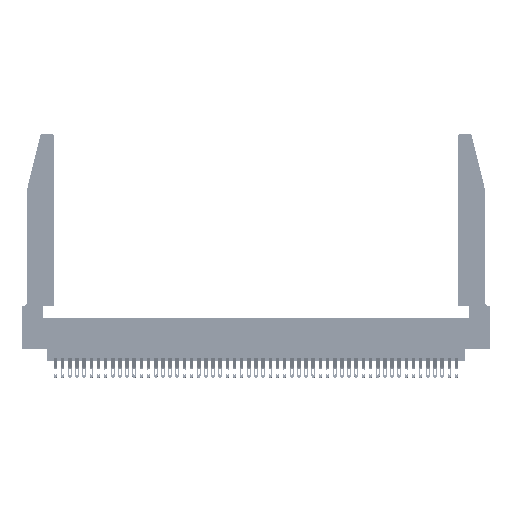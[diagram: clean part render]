
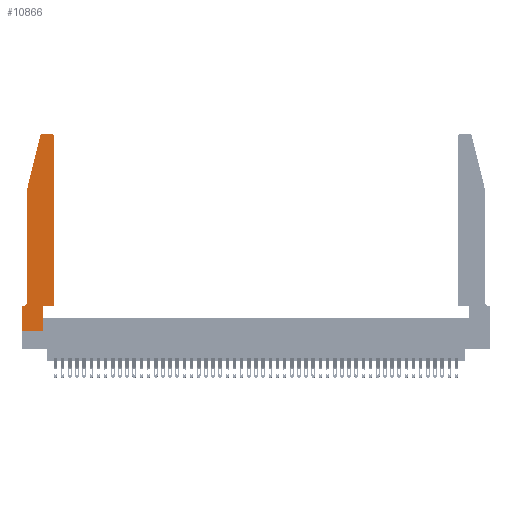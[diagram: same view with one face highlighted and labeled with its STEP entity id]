
A CAD part, top view. The second image highlights one B-rep face of the part: STEP entity #10866.
In plain terms, the highlighted planar face has unit normal (0, 0, 1).
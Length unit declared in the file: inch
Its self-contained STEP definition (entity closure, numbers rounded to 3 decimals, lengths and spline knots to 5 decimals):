
#9 = VERTEX_POINT ( 'NONE', #42469 ) ;
#34 = DIRECTION ( 'NONE',  ( 0., 0., -1. ) ) ;
#800 = LINE ( 'NONE', #43074, #20768 ) ;
#1021 = DIRECTION ( 'NONE',  ( 0., 1., 0. ) ) ;
#2736 = ORIENTED_EDGE ( 'NONE', *, *, #31449, .T. ) ;
#3164 = VERTEX_POINT ( 'NONE', #34432 ) ;
#3414 = VECTOR ( 'NONE', #1021, 39.37008 ) ;
#4061 = DIRECTION ( 'NONE',  ( 1., 0., 0. ) ) ;
#5102 = ORIENTED_EDGE ( 'NONE', *, *, #32296, .T. ) ;
#5123 = LINE ( 'NONE', #26429, #23848 ) ;
#5332 = VECTOR ( 'NONE', #27551, 39.37008 ) ;
#5709 = DIRECTION ( 'NONE',  ( 0., 0., 1. ) ) ;
#5745 = PLANE ( 'NONE',  #34677 ) ;
#5918 = DIRECTION ( 'NONE',  ( -1., 0., 0. ) ) ;
#5928 = CARTESIAN_POINT ( 'NONE',  ( 0.4205, 2.72, 0.37 ) ) ;
#7140 = ORIENTED_EDGE ( 'NONE', *, *, #41401, .T. ) ;
#7609 = EDGE_CURVE ( 'NONE', #45134, #28492, #46839, .T. ) ;
#7830 = CARTESIAN_POINT ( 'NONE',  ( 0., 0., 0.37 ) ) ;
#8157 = EDGE_CURVE ( 'NONE', #40730, #31751, #12805, .T. ) ;
#8918 = CARTESIAN_POINT ( 'NONE',  ( 0.2865, 0.35, 0.37 ) ) ;
#9130 = ORIENTED_EDGE ( 'NONE', *, *, #18466, .T. ) ;
#9181 = CARTESIAN_POINT ( 'NONE',  ( 0.4505, 0.35, 0.37 ) ) ;
#9729 = DIRECTION ( 'NONE',  ( 1., 0., 0. ) ) ;
#10556 = LINE ( 'NONE', #36836, #29129 ) ;
#10817 = ORIENTED_EDGE ( 'NONE', *, *, #7609, .T. ) ;
#10866 = ADVANCED_FACE ( 'NONE', ( #25432 ), #5745, .T. ) ;
#11307 = CARTESIAN_POINT ( 'NONE',  ( 0.0055, 0.35, 0.37 ) ) ;
#12038 = CARTESIAN_POINT ( 'NONE',  ( 0.284, 2.75, 0.37 ) ) ;
#12184 = ORIENTED_EDGE ( 'NONE', *, *, #20235, .T. ) ;
#12805 = LINE ( 'NONE', #9181, #42186 ) ;
#13967 = CIRCLE ( 'NONE', #18589, 0.03 ) ;
#13994 = EDGE_CURVE ( 'NONE', #31751, #43230, #24450, .T. ) ;
#14331 = ORIENTED_EDGE ( 'NONE', *, *, #13994, .T. ) ;
#15567 = LINE ( 'NONE', #7830, #44855 ) ;
#16008 = CARTESIAN_POINT ( 'NONE',  ( 0.4505, 0.35, 0.37 ) ) ;
#16404 = VECTOR ( 'NONE', #5918, 39.37008 ) ;
#16505 = ORIENTED_EDGE ( 'NONE', *, *, #47324, .T. ) ;
#16528 = ORIENTED_EDGE ( 'NONE', *, *, #45774, .T. ) ;
#16894 = CARTESIAN_POINT ( 'NONE',  ( 0.4505, 2.72, 0.37 ) ) ;
#17083 = DIRECTION ( 'NONE',  ( 0., 0., 1. ) ) ;
#17480 = ORIENTED_EDGE ( 'NONE', *, *, #44510, .T. ) ;
#18466 = EDGE_CURVE ( 'NONE', #9, #19691, #25765, .T. ) ;
#18589 = AXIS2_PLACEMENT_3D ( 'NONE', #28015, #5709, #31648 ) ;
#19151 = DIRECTION ( 'NONE',  ( 0., -1., 0. ) ) ;
#19691 = VERTEX_POINT ( 'NONE', #11307 ) ;
#20235 = EDGE_CURVE ( 'NONE', #24052, #40881, #15567, .T. ) ;
#20768 = VECTOR ( 'NONE', #21163, 39.37008 ) ;
#20846 = CARTESIAN_POINT ( 'NONE',  ( 0., 0., 0.37 ) ) ;
#20942 = CARTESIAN_POINT ( 'NONE',  ( 0.4205, 2.75, 0.37 ) ) ;
#21163 = DIRECTION ( 'NONE',  ( 0., 1., 0. ) ) ;
#21602 = CARTESIAN_POINT ( 'NONE',  ( 0.2865, 0., 0.37 ) ) ;
#22016 = AXIS2_PLACEMENT_3D ( 'NONE', #22506, #34, #26226 ) ;
#22506 = CARTESIAN_POINT ( 'NONE',  ( 0.0055, 0.42, 0.37 ) ) ;
#23296 = AXIS2_PLACEMENT_3D ( 'NONE', #5928, #31893, #9729 ) ;
#23626 = CARTESIAN_POINT ( 'NONE',  ( 0., 0.35, 0.37 ) ) ;
#23848 = VECTOR ( 'NONE', #4061, 39.37008 ) ;
#23877 = CARTESIAN_POINT ( 'NONE',  ( 0.0755, 2., 0.37 ) ) ;
#24052 = VERTEX_POINT ( 'NONE', #23626 ) ;
#24055 = LINE ( 'NONE', #23877, #5332 ) ;
#24450 = LINE ( 'NONE', #16008, #3414 ) ;
#25432 = FACE_OUTER_BOUND ( 'NONE', #29331, .T. ) ;
#25765 = CIRCLE ( 'NONE', #22016, 0.07 ) ;
#26226 = DIRECTION ( 'NONE',  ( -1., 0., 0. ) ) ;
#26429 = CARTESIAN_POINT ( 'NONE',  ( 0., 0., 0.37 ) ) ;
#27551 = DIRECTION ( 'NONE',  ( 0., -1., 0. ) ) ;
#27660 = ORIENTED_EDGE ( 'NONE', *, *, #43248, .T. ) ;
#28015 = CARTESIAN_POINT ( 'NONE',  ( 0.284, 2.72, 0.37 ) ) ;
#28492 = VERTEX_POINT ( 'NONE', #12038 ) ;
#29129 = VECTOR ( 'NONE', #29502, 39.37008 ) ;
#29331 = EDGE_LOOP ( 'NONE', ( #10817, #27660, #16528, #7140, #9130, #16505, #12184, #5102, #17480, #32239, #14331, #2736 ) ) ;
#29404 = VERTEX_POINT ( 'NONE', #21602 ) ;
#29502 = DIRECTION ( 'NONE',  ( -1., 0., 0. ) ) ;
#29649 = CARTESIAN_POINT ( 'NONE',  ( 0.4505, 0.35, 0.37 ) ) ;
#31340 = DIRECTION ( 'NONE',  ( 1., 0., 0. ) ) ;
#31449 = EDGE_CURVE ( 'NONE', #43230, #45134, #34121, .T. ) ;
#31648 = DIRECTION ( 'NONE',  ( 1., 0., 0. ) ) ;
#31751 = VERTEX_POINT ( 'NONE', #29649 ) ;
#31893 = DIRECTION ( 'NONE',  ( 0., 0., 1. ) ) ;
#32239 = ORIENTED_EDGE ( 'NONE', *, *, #8157, .T. ) ;
#32296 = EDGE_CURVE ( 'NONE', #40881, #29404, #5123, .T. ) ;
#33809 = VECTOR ( 'NONE', #38978, 39.37008 ) ;
#34121 = CIRCLE ( 'NONE', #23296, 0.03 ) ;
#34432 = CARTESIAN_POINT ( 'NONE',  ( 0.25487, 2.72718, 0.37 ) ) ;
#34642 = VERTEX_POINT ( 'NONE', #34869 ) ;
#34677 = AXIS2_PLACEMENT_3D ( 'NONE', #42400, #17083, #42735 ) ;
#34869 = CARTESIAN_POINT ( 'NONE',  ( 0.0755, 2., 0.37 ) ) ;
#36836 = CARTESIAN_POINT ( 'NONE',  ( 0.0755, 0.35, 0.37 ) ) ;
#38978 = DIRECTION ( 'NONE',  ( -0.239, -0.971, 0. ) ) ;
#39234 = CARTESIAN_POINT ( 'NONE',  ( 0.2605, 2.75, 0.37 ) ) ;
#40730 = VERTEX_POINT ( 'NONE', #8918 ) ;
#40881 = VERTEX_POINT ( 'NONE', #20846 ) ;
#41401 = EDGE_CURVE ( 'NONE', #34642, #9, #24055, .T. ) ;
#42186 = VECTOR ( 'NONE', #31340, 39.37008 ) ;
#42400 = CARTESIAN_POINT ( 'NONE',  ( 0., 0.35, 0.37 ) ) ;
#42469 = CARTESIAN_POINT ( 'NONE',  ( 0.0755, 0.42, 0.37 ) ) ;
#42649 = CARTESIAN_POINT ( 'NONE',  ( 0.0755, 2., 0.37 ) ) ;
#42735 = DIRECTION ( 'NONE',  ( 1., 0., 0. ) ) ;
#43074 = CARTESIAN_POINT ( 'NONE',  ( 0.2865, 0.35, 0.37 ) ) ;
#43230 = VERTEX_POINT ( 'NONE', #16894 ) ;
#43248 = EDGE_CURVE ( 'NONE', #28492, #3164, #13967, .T. ) ;
#43565 = LINE ( 'NONE', #42649, #33809 ) ;
#44510 = EDGE_CURVE ( 'NONE', #29404, #40730, #800, .T. ) ;
#44855 = VECTOR ( 'NONE', #19151, 39.37008 ) ;
#45134 = VERTEX_POINT ( 'NONE', #20942 ) ;
#45774 = EDGE_CURVE ( 'NONE', #3164, #34642, #43565, .T. ) ;
#46839 = LINE ( 'NONE', #39234, #16404 ) ;
#47324 = EDGE_CURVE ( 'NONE', #19691, #24052, #10556, .T. ) ;
